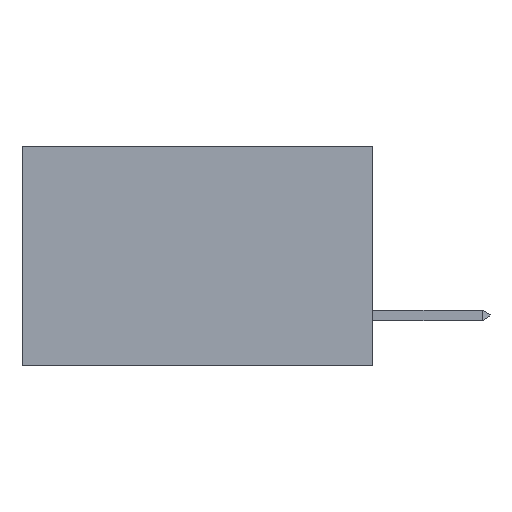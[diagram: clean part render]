
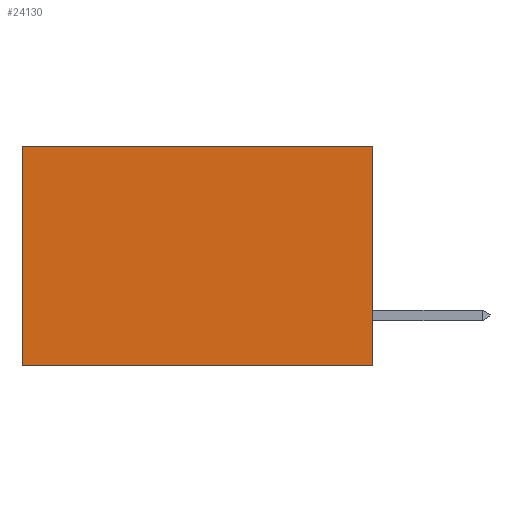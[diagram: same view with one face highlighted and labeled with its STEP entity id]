
A CAD part, left-side view. The second image highlights one B-rep face of the part: STEP entity #24130.
In plain terms, the highlighted planar face has unit normal (-1, 0, 0).
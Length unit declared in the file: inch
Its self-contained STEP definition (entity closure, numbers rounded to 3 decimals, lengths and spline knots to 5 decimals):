
#241 = CARTESIAN_POINT ( 'NONE',  ( 0.277, 0., 0. ) ) ;
#3816 = VECTOR ( 'NONE', #29320, 39.37008 ) ;
#4077 = CARTESIAN_POINT ( 'NONE',  ( 0.277, 0., -0.37 ) ) ;
#4850 = PLANE ( 'NONE',  #8355 ) ;
#5423 = CARTESIAN_POINT ( 'NONE',  ( 0.277, 0.59, 0. ) ) ;
#6126 = VECTOR ( 'NONE', #20302, 39.37008 ) ;
#6879 = VERTEX_POINT ( 'NONE', #241 ) ;
#7243 = CARTESIAN_POINT ( 'NONE',  ( 0.277, 0., 0. ) ) ;
#7286 = DIRECTION ( 'NONE',  ( 0., 0., -1. ) ) ;
#7718 = ORIENTED_EDGE ( 'NONE', *, *, #27147, .T. ) ;
#8355 = AXIS2_PLACEMENT_3D ( 'NONE', #14615, #21942, #7286 ) ;
#8422 = EDGE_CURVE ( 'NONE', #25965, #20704, #31235, .T. ) ;
#9799 = VECTOR ( 'NONE', #22217, 39.37008 ) ;
#11483 = EDGE_CURVE ( 'NONE', #29659, #20704, #29220, .T. ) ;
#12653 = EDGE_LOOP ( 'NONE', ( #26491, #29701, #17554, #7718 ) ) ;
#13834 = LINE ( 'NONE', #7243, #26013 ) ;
#14615 = CARTESIAN_POINT ( 'NONE',  ( 0.277, 0., -0.37 ) ) ;
#17126 = DIRECTION ( 'NONE',  ( 0., 1., 0. ) ) ;
#17554 = ORIENTED_EDGE ( 'NONE', *, *, #18620, .F. ) ;
#18620 = EDGE_CURVE ( 'NONE', #6879, #29659, #23306, .T. ) ;
#19417 = FACE_OUTER_BOUND ( 'NONE', #12653, .T. ) ;
#20092 = CARTESIAN_POINT ( 'NONE',  ( 0.277, 0.59, -0.37 ) ) ;
#20302 = DIRECTION ( 'NONE',  ( 0., 0., -1. ) ) ;
#20704 = VERTEX_POINT ( 'NONE', #22989 ) ;
#21942 = DIRECTION ( 'NONE',  ( 1., 0., 0. ) ) ;
#22217 = DIRECTION ( 'NONE',  ( 0., 1., 0. ) ) ;
#22989 = CARTESIAN_POINT ( 'NONE',  ( 0.277, 0.59, -0.37 ) ) ;
#23306 = LINE ( 'NONE', #26886, #3816 ) ;
#24130 = ADVANCED_FACE ( 'NONE', ( #19417 ), #4850, .F. ) ;
#24679 = CARTESIAN_POINT ( 'NONE',  ( 0.277, 0., -0.37 ) ) ;
#25965 = VERTEX_POINT ( 'NONE', #5423 ) ;
#26013 = VECTOR ( 'NONE', #17126, 39.37008 ) ;
#26491 = ORIENTED_EDGE ( 'NONE', *, *, #8422, .T. ) ;
#26886 = CARTESIAN_POINT ( 'NONE',  ( 0.277, 0., -0.37 ) ) ;
#27147 = EDGE_CURVE ( 'NONE', #6879, #25965, #13834, .T. ) ;
#29220 = LINE ( 'NONE', #24679, #9799 ) ;
#29320 = DIRECTION ( 'NONE',  ( 0., 0., -1. ) ) ;
#29659 = VERTEX_POINT ( 'NONE', #4077 ) ;
#29701 = ORIENTED_EDGE ( 'NONE', *, *, #11483, .F. ) ;
#31235 = LINE ( 'NONE', #20092, #6126 ) ;
